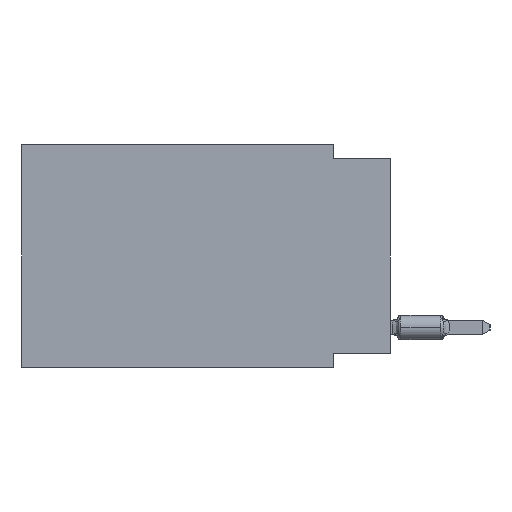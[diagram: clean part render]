
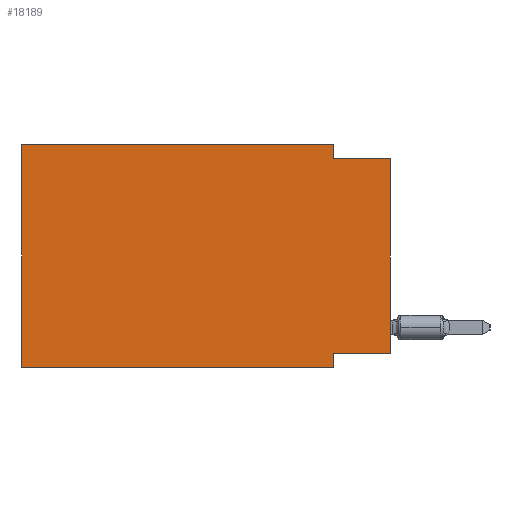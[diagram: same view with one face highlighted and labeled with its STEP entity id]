
A CAD part, left-side view. The second image highlights one B-rep face of the part: STEP entity #18189.
In plain terms, the highlighted planar face has unit normal (-1, 0, 0).
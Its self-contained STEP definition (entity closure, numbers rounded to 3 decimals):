
#256 = LINE ( 'NONE', #30164, #9616 ) ;
#820 = CARTESIAN_POINT ( 'NONE',  ( 0., 0., 0. ) ) ;
#985 = EDGE_CURVE ( 'NONE', #13221, #21514, #31589, .T. ) ;
#1485 = VECTOR ( 'NONE', #25224, 1000. ) ;
#2080 = VERTEX_POINT ( 'NONE', #8341 ) ;
#2258 = CARTESIAN_POINT ( 'NONE',  ( 0., 0., -0.635 ) ) ;
#2614 = EDGE_LOOP ( 'NONE', ( #6821, #11425, #23165, #6650, #26309, #21289, #21939, #24340 ) ) ;
#3597 = VECTOR ( 'NONE', #9447, 1000. ) ;
#4529 = DIRECTION ( 'NONE',  ( 0., -1., 0. ) ) ;
#4600 = CARTESIAN_POINT ( 'NONE',  ( 0., 2.54, -9.271 ) ) ;
#6650 = ORIENTED_EDGE ( 'NONE', *, *, #20149, .F. ) ;
#6821 = ORIENTED_EDGE ( 'NONE', *, *, #19112, .T. ) ;
#7713 = DIRECTION ( 'NONE',  ( 0., 1., 0. ) ) ;
#8178 = VECTOR ( 'NONE', #9304, 1000. ) ;
#8341 = CARTESIAN_POINT ( 'NONE',  ( 0., 2.54, 0. ) ) ;
#8414 = CARTESIAN_POINT ( 'NONE',  ( 0., 16.383, -9.906 ) ) ;
#8451 = DIRECTION ( 'NONE',  ( 0., 0., -1. ) ) ;
#9304 = DIRECTION ( 'NONE',  ( 0., -1., 0. ) ) ;
#9440 = DIRECTION ( 'NONE',  ( 0., 0., 1. ) ) ;
#9447 = DIRECTION ( 'NONE',  ( 0., 0., -1. ) ) ;
#9616 = VECTOR ( 'NONE', #7713, 1000. ) ;
#10671 = EDGE_CURVE ( 'NONE', #2080, #18238, #11703, .T. ) ;
#10962 = CARTESIAN_POINT ( 'NONE',  ( 0., 16.383, 0. ) ) ;
#11425 = ORIENTED_EDGE ( 'NONE', *, *, #17854, .F. ) ;
#11703 = LINE ( 'NONE', #31924, #3597 ) ;
#11795 = LINE ( 'NONE', #2258, #17939 ) ;
#13221 = VERTEX_POINT ( 'NONE', #19813 ) ;
#13239 = EDGE_CURVE ( 'NONE', #24002, #25682, #256, .T. ) ;
#13393 = FACE_OUTER_BOUND ( 'NONE', #2614, .T. ) ;
#14332 = AXIS2_PLACEMENT_3D ( 'NONE', #10962, #20814, #30689 ) ;
#14447 = CARTESIAN_POINT ( 'NONE',  ( 0., 16.383, 0. ) ) ;
#14911 = VERTEX_POINT ( 'NONE', #25566 ) ;
#17837 = CARTESIAN_POINT ( 'NONE',  ( 0., 16.383, 0. ) ) ;
#17854 = EDGE_CURVE ( 'NONE', #18238, #14911, #11795, .T. ) ;
#17939 = VECTOR ( 'NONE', #4529, 1000. ) ;
#18189 = ADVANCED_FACE ( 'NONE', ( #13393 ), #23261, .F. ) ;
#18238 = VERTEX_POINT ( 'NONE', #19342 ) ;
#18434 = LINE ( 'NONE', #820, #1485 ) ;
#18517 = VERTEX_POINT ( 'NONE', #31632 ) ;
#19112 = EDGE_CURVE ( 'NONE', #24002, #14911, #18434, .T. ) ;
#19222 = VECTOR ( 'NONE', #8451, 1000. ) ;
#19342 = CARTESIAN_POINT ( 'NONE',  ( 0., 2.54, -0.635 ) ) ;
#19813 = CARTESIAN_POINT ( 'NONE',  ( 0., 16.383, -9.906 ) ) ;
#20149 = EDGE_CURVE ( 'NONE', #21514, #2080, #27215, .T. ) ;
#20814 = DIRECTION ( 'NONE',  ( 1., 0., 0. ) ) ;
#21289 = ORIENTED_EDGE ( 'NONE', *, *, #23564, .T. ) ;
#21514 = VERTEX_POINT ( 'NONE', #17837 ) ;
#21909 = VECTOR ( 'NONE', #9440, 1000. ) ;
#21939 = ORIENTED_EDGE ( 'NONE', *, *, #24370, .F. ) ;
#22060 = CARTESIAN_POINT ( 'NONE',  ( 0., 16.383, 0. ) ) ;
#23165 = ORIENTED_EDGE ( 'NONE', *, *, #10671, .F. ) ;
#23261 = PLANE ( 'NONE',  #14332 ) ;
#23280 = DIRECTION ( 'NONE',  ( 0., -1., 0. ) ) ;
#23564 = EDGE_CURVE ( 'NONE', #13221, #18517, #28442, .T. ) ;
#24002 = VERTEX_POINT ( 'NONE', #30518 ) ;
#24340 = ORIENTED_EDGE ( 'NONE', *, *, #13239, .F. ) ;
#24370 = EDGE_CURVE ( 'NONE', #25682, #18517, #26045, .T. ) ;
#25224 = DIRECTION ( 'NONE',  ( 0., 0., 1. ) ) ;
#25566 = CARTESIAN_POINT ( 'NONE',  ( 0., 0., -0.635 ) ) ;
#25682 = VERTEX_POINT ( 'NONE', #4600 ) ;
#26045 = LINE ( 'NONE', #28157, #19222 ) ;
#26309 = ORIENTED_EDGE ( 'NONE', *, *, #985, .F. ) ;
#27179 = VECTOR ( 'NONE', #23280, 1000. ) ;
#27215 = LINE ( 'NONE', #22060, #8178 ) ;
#28157 = CARTESIAN_POINT ( 'NONE',  ( 0., 2.54, -9.906 ) ) ;
#28442 = LINE ( 'NONE', #8414, #27179 ) ;
#30164 = CARTESIAN_POINT ( 'NONE',  ( 0., 0., -9.271 ) ) ;
#30518 = CARTESIAN_POINT ( 'NONE',  ( 0., 0., -9.271 ) ) ;
#30689 = DIRECTION ( 'NONE',  ( 0., 0., -1. ) ) ;
#31589 = LINE ( 'NONE', #14447, #21909 ) ;
#31632 = CARTESIAN_POINT ( 'NONE',  ( 0., 2.54, -9.906 ) ) ;
#31924 = CARTESIAN_POINT ( 'NONE',  ( 0., 2.54, 0. ) ) ;
